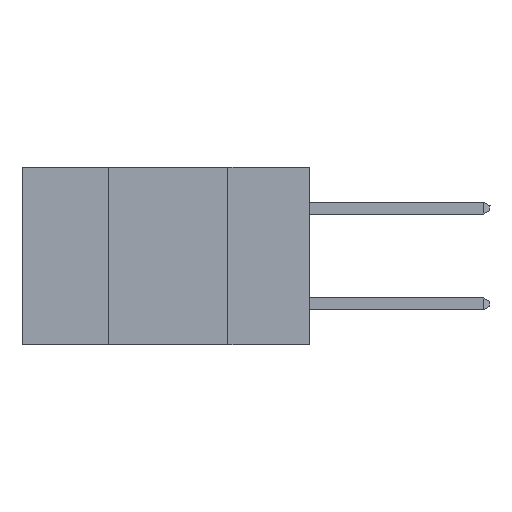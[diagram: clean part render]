
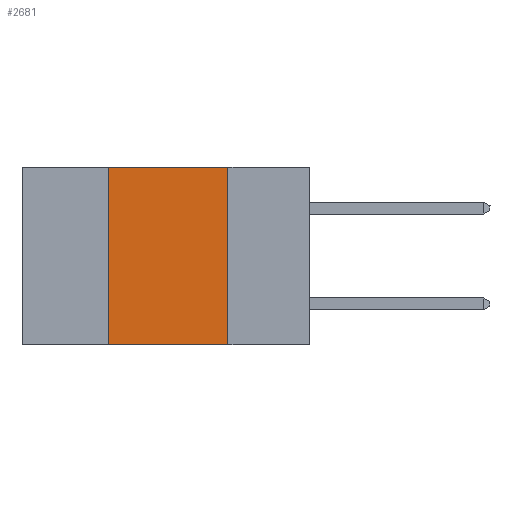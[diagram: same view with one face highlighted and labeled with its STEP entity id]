
A CAD part, left-side view. The second image highlights one B-rep face of the part: STEP entity #2681.
In plain terms, the highlighted planar face has unit normal (-1, 0, 0).
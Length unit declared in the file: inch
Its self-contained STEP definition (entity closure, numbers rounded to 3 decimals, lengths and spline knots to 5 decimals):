
#28 = VECTOR ( 'NONE', #5792, 39.37008 ) ;
#59 = VECTOR ( 'NONE', #1357, 39.37008 ) ;
#322 = LINE ( 'NONE', #10507, #7020 ) ;
#446 = ORIENTED_EDGE ( 'NONE', *, *, #13594, .T. ) ;
#716 = EDGE_CURVE ( 'NONE', #8760, #3975, #3640, .T. ) ;
#862 = DIRECTION ( 'NONE',  ( 0., -1., 0. ) ) ;
#1025 = CARTESIAN_POINT ( 'NONE',  ( 0., 0.6, 0. ) ) ;
#1087 = ORIENTED_EDGE ( 'NONE', *, *, #716, .F. ) ;
#1357 = DIRECTION ( 'NONE',  ( 0., 0., -1. ) ) ;
#2472 = LINE ( 'NONE', #1025, #7489 ) ;
#2681 = ADVANCED_FACE ( 'NONE', ( #6748 ), #6829, .F. ) ;
#3186 = DIRECTION ( 'NONE',  ( 0., 0., -1. ) ) ;
#3544 = EDGE_CURVE ( 'NONE', #12753, #6150, #13298, .T. ) ;
#3640 = LINE ( 'NONE', #4708, #59 ) ;
#3975 = VERTEX_POINT ( 'NONE', #12307 ) ;
#4342 = DIRECTION ( 'NONE',  ( 1., 0., 0. ) ) ;
#4708 = CARTESIAN_POINT ( 'NONE',  ( 0., 0.17, 0. ) ) ;
#5189 = CARTESIAN_POINT ( 'NONE',  ( 0., 0.42, 0. ) ) ;
#5792 = DIRECTION ( 'NONE',  ( 0., 0., 1. ) ) ;
#6150 = VERTEX_POINT ( 'NONE', #5189 ) ;
#6604 = CARTESIAN_POINT ( 'NONE',  ( 0., 0.6, 0. ) ) ;
#6748 = FACE_OUTER_BOUND ( 'NONE', #8506, .T. ) ;
#6829 = PLANE ( 'NONE',  #7922 ) ;
#7020 = VECTOR ( 'NONE', #10653, 39.37008 ) ;
#7433 = EDGE_CURVE ( 'NONE', #6150, #8760, #2472, .T. ) ;
#7489 = VECTOR ( 'NONE', #862, 39.37008 ) ;
#7922 = AXIS2_PLACEMENT_3D ( 'NONE', #6604, #4342, #3186 ) ;
#8375 = CARTESIAN_POINT ( 'NONE',  ( 0., 0.42, 0. ) ) ;
#8506 = EDGE_LOOP ( 'NONE', ( #1087, #10253, #11700, #446 ) ) ;
#8760 = VERTEX_POINT ( 'NONE', #13717 ) ;
#9161 = CARTESIAN_POINT ( 'NONE',  ( 0., 0.42, -0.37 ) ) ;
#10253 = ORIENTED_EDGE ( 'NONE', *, *, #7433, .F. ) ;
#10507 = CARTESIAN_POINT ( 'NONE',  ( 0., 0.6, -0.37 ) ) ;
#10653 = DIRECTION ( 'NONE',  ( 0., -1., 0. ) ) ;
#11700 = ORIENTED_EDGE ( 'NONE', *, *, #3544, .F. ) ;
#12307 = CARTESIAN_POINT ( 'NONE',  ( 0., 0.17, -0.37 ) ) ;
#12753 = VERTEX_POINT ( 'NONE', #9161 ) ;
#13298 = LINE ( 'NONE', #8375, #28 ) ;
#13594 = EDGE_CURVE ( 'NONE', #12753, #3975, #322, .T. ) ;
#13717 = CARTESIAN_POINT ( 'NONE',  ( 0., 0.17, 0. ) ) ;
